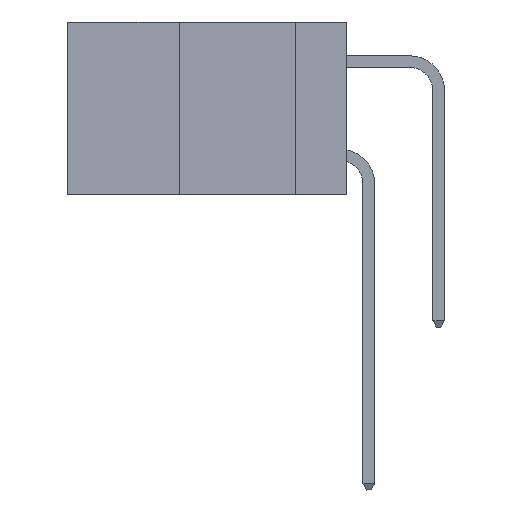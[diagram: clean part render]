
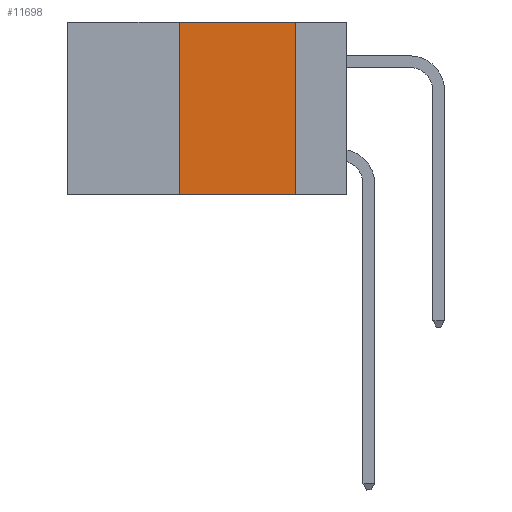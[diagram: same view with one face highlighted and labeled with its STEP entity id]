
A CAD part, left-side view. The second image highlights one B-rep face of the part: STEP entity #11698.
In plain terms, the highlighted planar face has unit normal (-1, 0, 0).
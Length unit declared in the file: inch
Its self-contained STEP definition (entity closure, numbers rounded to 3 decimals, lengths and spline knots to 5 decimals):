
#839 = AXIS2_PLACEMENT_3D ( 'NONE', #13085, #13008, #3158 ) ;
#1054 = CARTESIAN_POINT ( 'NONE',  ( 0., 0.11, -0.37 ) ) ;
#1552 = EDGE_CURVE ( 'NONE', #2695, #13069, #17223, .T. ) ;
#1978 = ORIENTED_EDGE ( 'NONE', *, *, #1552, .F. ) ;
#2695 = VERTEX_POINT ( 'NONE', #18717 ) ;
#2931 = DIRECTION ( 'NONE',  ( 0., -1., 0. ) ) ;
#3158 = DIRECTION ( 'NONE',  ( 0., 0., -1. ) ) ;
#4642 = CARTESIAN_POINT ( 'NONE',  ( 0., 0.36, 0. ) ) ;
#4706 = VECTOR ( 'NONE', #14639, 39.37008 ) ;
#5683 = EDGE_CURVE ( 'NONE', #22025, #21669, #7860, .T. ) ;
#6051 = CARTESIAN_POINT ( 'NONE',  ( 0., 0.11, 0. ) ) ;
#7860 = LINE ( 'NONE', #19542, #24554 ) ;
#9254 = EDGE_CURVE ( 'NONE', #21669, #2695, #11056, .T. ) ;
#9295 = PLANE ( 'NONE',  #839 ) ;
#10307 = FACE_OUTER_BOUND ( 'NONE', #19049, .T. ) ;
#10735 = CARTESIAN_POINT ( 'NONE',  ( 0., 0.6, 0. ) ) ;
#10963 = ORIENTED_EDGE ( 'NONE', *, *, #20453, .T. ) ;
#11056 = LINE ( 'NONE', #10735, #4706 ) ;
#11698 = ADVANCED_FACE ( 'NONE', ( #10307 ), #9295, .F. ) ;
#11998 = VECTOR ( 'NONE', #2931, 39.37008 ) ;
#12040 = VECTOR ( 'NONE', #14205, 39.37008 ) ;
#13008 = DIRECTION ( 'NONE',  ( 1., 0., 0. ) ) ;
#13069 = VERTEX_POINT ( 'NONE', #1054 ) ;
#13085 = CARTESIAN_POINT ( 'NONE',  ( 0., 0.6, 0. ) ) ;
#14205 = DIRECTION ( 'NONE',  ( 0., 0., -1. ) ) ;
#14639 = DIRECTION ( 'NONE',  ( 0., -1., 0. ) ) ;
#14989 = ORIENTED_EDGE ( 'NONE', *, *, #5683, .F. ) ;
#16185 = ORIENTED_EDGE ( 'NONE', *, *, #9254, .F. ) ;
#17185 = LINE ( 'NONE', #23965, #11998 ) ;
#17223 = LINE ( 'NONE', #6051, #12040 ) ;
#18717 = CARTESIAN_POINT ( 'NONE',  ( 0., 0.11, 0. ) ) ;
#19049 = EDGE_LOOP ( 'NONE', ( #1978, #16185, #14989, #10963 ) ) ;
#19542 = CARTESIAN_POINT ( 'NONE',  ( 0., 0.36, 0. ) ) ;
#19948 = DIRECTION ( 'NONE',  ( 0., 0., 1. ) ) ;
#20453 = EDGE_CURVE ( 'NONE', #22025, #13069, #17185, .T. ) ;
#21669 = VERTEX_POINT ( 'NONE', #4642 ) ;
#22025 = VERTEX_POINT ( 'NONE', #22634 ) ;
#22634 = CARTESIAN_POINT ( 'NONE',  ( 0., 0.36, -0.37 ) ) ;
#23965 = CARTESIAN_POINT ( 'NONE',  ( 0., 0.6, -0.37 ) ) ;
#24554 = VECTOR ( 'NONE', #19948, 39.37008 ) ;
